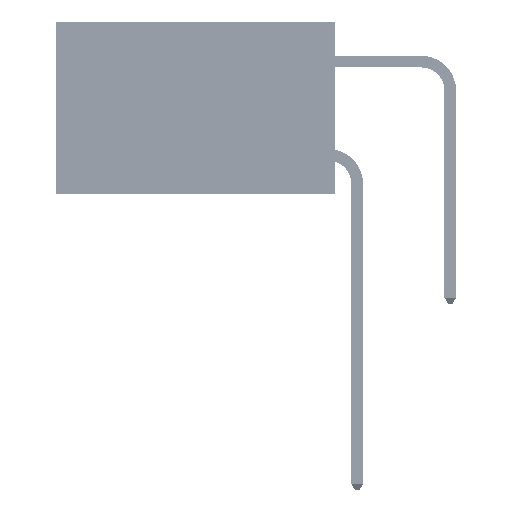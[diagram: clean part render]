
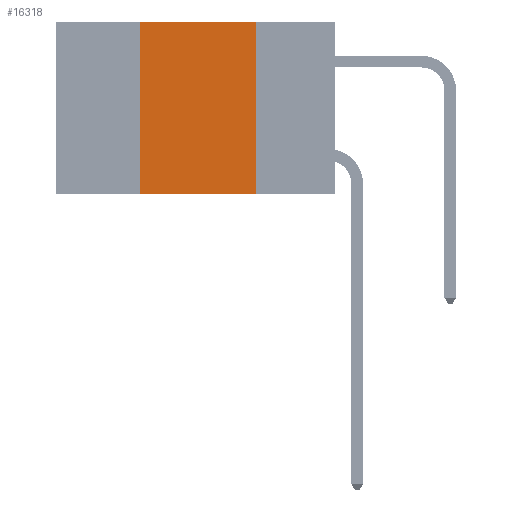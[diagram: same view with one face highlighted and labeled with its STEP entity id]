
A CAD part, left-side view. The second image highlights one B-rep face of the part: STEP entity #16318.
In plain terms, the highlighted planar face has unit normal (-1, 0, 0).
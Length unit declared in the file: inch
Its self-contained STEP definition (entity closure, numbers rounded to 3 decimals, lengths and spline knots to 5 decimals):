
#1836 = LINE ( 'NONE', #39952, #29317 ) ;
#3461 = EDGE_CURVE ( 'NONE', #8293, #30450, #1836, .T. ) ;
#3924 = LINE ( 'NONE', #13436, #26486 ) ;
#4320 = ORIENTED_EDGE ( 'NONE', *, *, #3461, .F. ) ;
#5003 = LINE ( 'NONE', #32645, #26972 ) ;
#5810 = EDGE_LOOP ( 'NONE', ( #4320, #47003, #30855, #44913 ) ) ;
#5990 = AXIS2_PLACEMENT_3D ( 'NONE', #23340, #38966, #15662 ) ;
#6096 = VERTEX_POINT ( 'NONE', #41299 ) ;
#6700 = EDGE_CURVE ( 'NONE', #6096, #14112, #37186, .T. ) ;
#6715 = CARTESIAN_POINT ( 'NONE',  ( 0., 0.17, 0. ) ) ;
#7855 = CARTESIAN_POINT ( 'NONE',  ( 0., 0.17, -0.37 ) ) ;
#8293 = VERTEX_POINT ( 'NONE', #6715 ) ;
#13436 = CARTESIAN_POINT ( 'NONE',  ( 0., 0.6, -0.37 ) ) ;
#14112 = VERTEX_POINT ( 'NONE', #25611 ) ;
#15498 = PLANE ( 'NONE',  #5990 ) ;
#15662 = DIRECTION ( 'NONE',  ( 0., 0., -1. ) ) ;
#16052 = FACE_OUTER_BOUND ( 'NONE', #5810, .T. ) ;
#16318 = ADVANCED_FACE ( 'NONE', ( #16052 ), #15498, .F. ) ;
#16959 = DIRECTION ( 'NONE',  ( 0., -1., 0. ) ) ;
#23340 = CARTESIAN_POINT ( 'NONE',  ( 0., 0.6, 0. ) ) ;
#25611 = CARTESIAN_POINT ( 'NONE',  ( 0., 0.42, 0. ) ) ;
#26486 = VECTOR ( 'NONE', #48437, 39.37008 ) ;
#26972 = VECTOR ( 'NONE', #16959, 39.37008 ) ;
#29317 = VECTOR ( 'NONE', #47776, 39.37008 ) ;
#30450 = VERTEX_POINT ( 'NONE', #7855 ) ;
#30855 = ORIENTED_EDGE ( 'NONE', *, *, #6700, .F. ) ;
#31755 = VECTOR ( 'NONE', #48532, 39.37008 ) ;
#32635 = CARTESIAN_POINT ( 'NONE',  ( 0., 0.42, 0. ) ) ;
#32645 = CARTESIAN_POINT ( 'NONE',  ( 0., 0.6, 0. ) ) ;
#33496 = EDGE_CURVE ( 'NONE', #14112, #8293, #5003, .T. ) ;
#37186 = LINE ( 'NONE', #32635, #31755 ) ;
#38966 = DIRECTION ( 'NONE',  ( 1., 0., 0. ) ) ;
#39952 = CARTESIAN_POINT ( 'NONE',  ( 0., 0.17, 0. ) ) ;
#41299 = CARTESIAN_POINT ( 'NONE',  ( 0., 0.42, -0.37 ) ) ;
#44913 = ORIENTED_EDGE ( 'NONE', *, *, #45367, .T. ) ;
#45367 = EDGE_CURVE ( 'NONE', #6096, #30450, #3924, .T. ) ;
#47003 = ORIENTED_EDGE ( 'NONE', *, *, #33496, .F. ) ;
#47776 = DIRECTION ( 'NONE',  ( 0., 0., -1. ) ) ;
#48437 = DIRECTION ( 'NONE',  ( 0., -1., 0. ) ) ;
#48532 = DIRECTION ( 'NONE',  ( 0., 0., 1. ) ) ;
